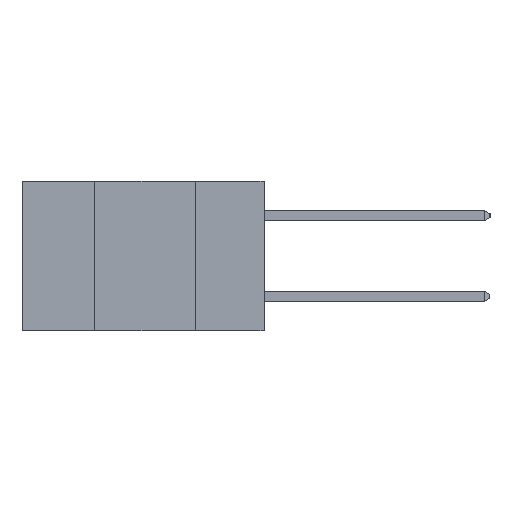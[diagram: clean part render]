
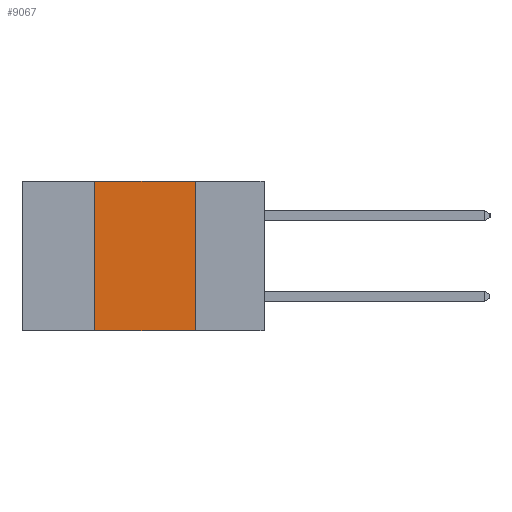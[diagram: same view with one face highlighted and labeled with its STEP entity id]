
A CAD part, left-side view. The second image highlights one B-rep face of the part: STEP entity #9067.
In plain terms, the highlighted planar face has unit normal (-1, 0, 0).
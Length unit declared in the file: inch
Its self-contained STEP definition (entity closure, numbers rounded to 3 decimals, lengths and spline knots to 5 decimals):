
#802 = VECTOR ( 'NONE', #14685, 39.37008 ) ;
#836 = VECTOR ( 'NONE', #2813, 39.37008 ) ;
#1492 = ORIENTED_EDGE ( 'NONE', *, *, #8718, .F. ) ;
#1515 = FACE_OUTER_BOUND ( 'NONE', #4413, .T. ) ;
#2736 = LINE ( 'NONE', #12989, #836 ) ;
#2813 = DIRECTION ( 'NONE',  ( 0., 0., -1. ) ) ;
#2897 = DIRECTION ( 'NONE',  ( 0., -1., 0. ) ) ;
#3333 = CARTESIAN_POINT ( 'NONE',  ( 0., 0.6, -0.37 ) ) ;
#3639 = LINE ( 'NONE', #12219, #4614 ) ;
#3868 = VERTEX_POINT ( 'NONE', #14233 ) ;
#3908 = AXIS2_PLACEMENT_3D ( 'NONE', #6941, #10410, #5807 ) ;
#4413 = EDGE_LOOP ( 'NONE', ( #8050, #12937, #1492, #9527 ) ) ;
#4614 = VECTOR ( 'NONE', #13049, 39.37008 ) ;
#4634 = VERTEX_POINT ( 'NONE', #4959 ) ;
#4865 = EDGE_CURVE ( 'NONE', #3868, #4634, #6229, .T. ) ;
#4959 = CARTESIAN_POINT ( 'NONE',  ( 0., 0.17, 0. ) ) ;
#5807 = DIRECTION ( 'NONE',  ( 0., 0., -1. ) ) ;
#6229 = LINE ( 'NONE', #10812, #11230 ) ;
#6941 = CARTESIAN_POINT ( 'NONE',  ( 0., 0.6, 0. ) ) ;
#7100 = CARTESIAN_POINT ( 'NONE',  ( 0., 0.17, -0.37 ) ) ;
#7369 = VERTEX_POINT ( 'NONE', #7100 ) ;
#8050 = ORIENTED_EDGE ( 'NONE', *, *, #11060, .F. ) ;
#8718 = EDGE_CURVE ( 'NONE', #13116, #3868, #3639, .T. ) ;
#9067 = ADVANCED_FACE ( 'NONE', ( #1515 ), #12742, .F. ) ;
#9527 = ORIENTED_EDGE ( 'NONE', *, *, #10047, .T. ) ;
#10047 = EDGE_CURVE ( 'NONE', #13116, #7369, #10122, .T. ) ;
#10122 = LINE ( 'NONE', #3333, #802 ) ;
#10410 = DIRECTION ( 'NONE',  ( 1., 0., 0. ) ) ;
#10812 = CARTESIAN_POINT ( 'NONE',  ( 0., 0.6, 0. ) ) ;
#11060 = EDGE_CURVE ( 'NONE', #4634, #7369, #2736, .T. ) ;
#11230 = VECTOR ( 'NONE', #2897, 39.37008 ) ;
#12219 = CARTESIAN_POINT ( 'NONE',  ( 0., 0.42, -0.37 ) ) ;
#12742 = PLANE ( 'NONE',  #3908 ) ;
#12937 = ORIENTED_EDGE ( 'NONE', *, *, #4865, .F. ) ;
#12989 = CARTESIAN_POINT ( 'NONE',  ( 0., 0.17, -0.37 ) ) ;
#13049 = DIRECTION ( 'NONE',  ( 0., 0., 1. ) ) ;
#13116 = VERTEX_POINT ( 'NONE', #13196 ) ;
#13196 = CARTESIAN_POINT ( 'NONE',  ( 0., 0.42, -0.37 ) ) ;
#14233 = CARTESIAN_POINT ( 'NONE',  ( 0., 0.42, 0. ) ) ;
#14685 = DIRECTION ( 'NONE',  ( 0., -1., 0. ) ) ;
